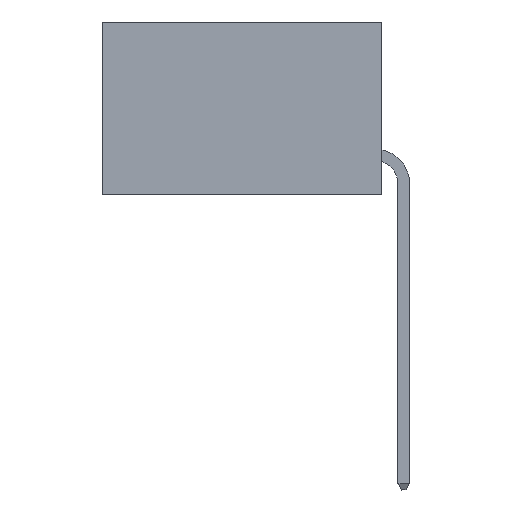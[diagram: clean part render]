
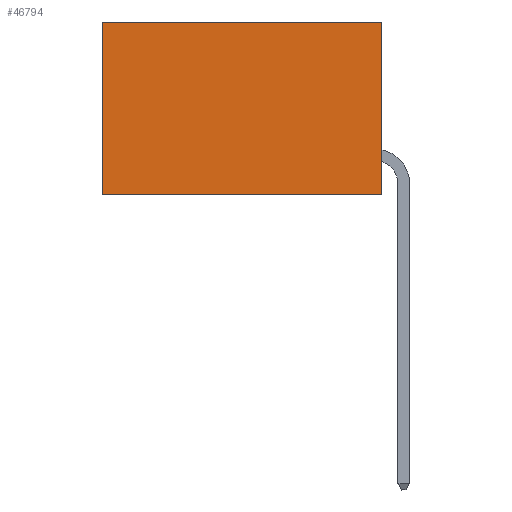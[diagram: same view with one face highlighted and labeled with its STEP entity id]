
A CAD part, left-side view. The second image highlights one B-rep face of the part: STEP entity #46794.
In plain terms, the highlighted planar face has unit normal (-1, 0, 0).
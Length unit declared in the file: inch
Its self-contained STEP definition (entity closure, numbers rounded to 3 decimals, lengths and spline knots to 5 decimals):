
#4882 = VERTEX_POINT ( 'NONE', #15865 ) ;
#7709 = CARTESIAN_POINT ( 'NONE',  ( 0.2875, 0.6, -0.37 ) ) ;
#8206 = CARTESIAN_POINT ( 'NONE',  ( 0.2875, 0., -0.37 ) ) ;
#9269 = EDGE_LOOP ( 'NONE', ( #24461, #21249, #26341, #39585 ) ) ;
#10924 = DIRECTION ( 'NONE',  ( 0., 1., 0. ) ) ;
#12590 = DIRECTION ( 'NONE',  ( 0., 0., -1. ) ) ;
#13424 = DIRECTION ( 'NONE',  ( 0., 1., 0. ) ) ;
#14822 = CARTESIAN_POINT ( 'NONE',  ( 0.2875, 0., 0. ) ) ;
#15154 = LINE ( 'NONE', #33982, #24171 ) ;
#15231 = CARTESIAN_POINT ( 'NONE',  ( 0.2875, 0.6, 0. ) ) ;
#15865 = CARTESIAN_POINT ( 'NONE',  ( 0.2875, 0., 0. ) ) ;
#15950 = PLANE ( 'NONE',  #29863 ) ;
#16325 = EDGE_CURVE ( 'NONE', #4882, #30828, #18777, .T. ) ;
#16971 = EDGE_CURVE ( 'NONE', #36390, #34733, #35619, .T. ) ;
#18610 = EDGE_CURVE ( 'NONE', #4882, #36390, #23314, .T. ) ;
#18777 = LINE ( 'NONE', #14822, #37546 ) ;
#21249 = ORIENTED_EDGE ( 'NONE', *, *, #24769, .F. ) ;
#23314 = LINE ( 'NONE', #42561, #27540 ) ;
#24171 = VECTOR ( 'NONE', #10924, 39.37008 ) ;
#24461 = ORIENTED_EDGE ( 'NONE', *, *, #16971, .T. ) ;
#24769 = EDGE_CURVE ( 'NONE', #30828, #34733, #15154, .T. ) ;
#26341 = ORIENTED_EDGE ( 'NONE', *, *, #16325, .F. ) ;
#27354 = DIRECTION ( 'NONE',  ( 0., 0., -1. ) ) ;
#27540 = VECTOR ( 'NONE', #13424, 39.37008 ) ;
#29863 = AXIS2_PLACEMENT_3D ( 'NONE', #43448, #43615, #12590 ) ;
#30346 = DIRECTION ( 'NONE',  ( 0., 0., -1. ) ) ;
#30828 = VERTEX_POINT ( 'NONE', #8206 ) ;
#33982 = CARTESIAN_POINT ( 'NONE',  ( 0.2875, 0., -0.37 ) ) ;
#34733 = VERTEX_POINT ( 'NONE', #7709 ) ;
#35619 = LINE ( 'NONE', #15231, #38628 ) ;
#36390 = VERTEX_POINT ( 'NONE', #37590 ) ;
#37546 = VECTOR ( 'NONE', #30346, 39.37008 ) ;
#37590 = CARTESIAN_POINT ( 'NONE',  ( 0.2875, 0.6, 0. ) ) ;
#38628 = VECTOR ( 'NONE', #27354, 39.37008 ) ;
#39585 = ORIENTED_EDGE ( 'NONE', *, *, #18610, .T. ) ;
#42561 = CARTESIAN_POINT ( 'NONE',  ( 0.2875, 0., 0. ) ) ;
#43448 = CARTESIAN_POINT ( 'NONE',  ( 0.2875, 0., 0. ) ) ;
#43615 = DIRECTION ( 'NONE',  ( 1., 0., 0. ) ) ;
#44960 = FACE_OUTER_BOUND ( 'NONE', #9269, .T. ) ;
#46794 = ADVANCED_FACE ( 'NONE', ( #44960 ), #15950, .F. ) ;
